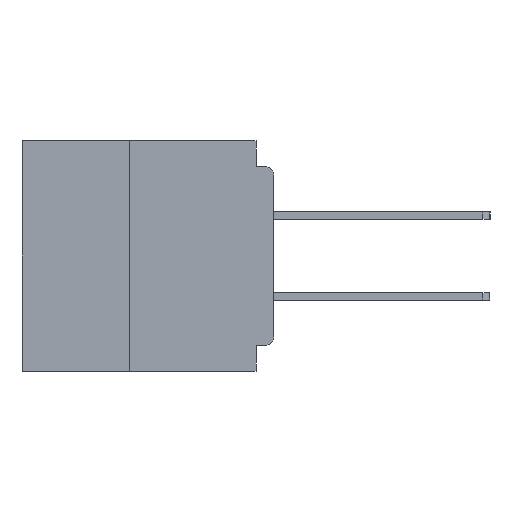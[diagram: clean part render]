
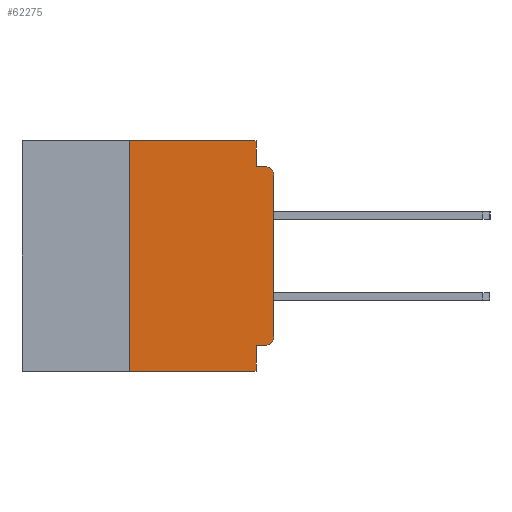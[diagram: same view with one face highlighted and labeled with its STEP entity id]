
A CAD part, left-side view. The second image highlights one B-rep face of the part: STEP entity #62275.
In plain terms, the highlighted planar face has unit normal (-1, 0, 0).
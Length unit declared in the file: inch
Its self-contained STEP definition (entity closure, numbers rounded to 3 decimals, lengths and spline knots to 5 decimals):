
#115 = LINE ( 'NONE', #27405, #37791 ) ;
#510 = CARTESIAN_POINT ( 'NONE',  ( 0., 0.031, 0. ) ) ;
#571 = VERTEX_POINT ( 'NONE', #45009 ) ;
#655 = DIRECTION ( 'NONE',  ( 0., 0., -1. ) ) ;
#2635 = ORIENTED_EDGE ( 'NONE', *, *, #33401, .T. ) ;
#2966 = CARTESIAN_POINT ( 'NONE',  ( 0., 0.437, 0. ) ) ;
#4892 = CARTESIAN_POINT ( 'NONE',  ( 0., 0.437, -0.4 ) ) ;
#5825 = EDGE_CURVE ( 'NONE', #58855, #42514, #52267, .T. ) ;
#7138 = VERTEX_POINT ( 'NONE', #64051 ) ;
#7331 = VECTOR ( 'NONE', #30076, 39.37008 ) ;
#7844 = CARTESIAN_POINT ( 'NONE',  ( 0., 0.015, -0.34 ) ) ;
#8143 = DIRECTION ( 'NONE',  ( 1., 0., 0. ) ) ;
#9761 = VECTOR ( 'NONE', #63482, 39.37008 ) ;
#10043 = DIRECTION ( 'NONE',  ( 0., -1., 0. ) ) ;
#12557 = CIRCLE ( 'NONE', #51729, 0.015 ) ;
#12967 = DIRECTION ( 'NONE',  ( 0., 0., -1. ) ) ;
#16704 = DIRECTION ( 'NONE',  ( -1., 0., 0. ) ) ;
#16877 = EDGE_CURVE ( 'NONE', #28326, #44976, #51607, .T. ) ;
#17175 = ORIENTED_EDGE ( 'NONE', *, *, #64541, .T. ) ;
#17293 = CARTESIAN_POINT ( 'NONE',  ( 0., 0., -0.355 ) ) ;
#17737 = DIRECTION ( 'NONE',  ( 0., -1., 0. ) ) ;
#18548 = CARTESIAN_POINT ( 'NONE',  ( 0., 0.015, -0.355 ) ) ;
#19412 = LINE ( 'NONE', #55279, #7331 ) ;
#19774 = EDGE_LOOP ( 'NONE', ( #2635, #41567, #21120, #51244, #49167, #52943, #44488, #63672, #28062, #17175 ) ) ;
#21120 = ORIENTED_EDGE ( 'NONE', *, *, #28034, .F. ) ;
#21624 = LINE ( 'NONE', #17293, #60496 ) ;
#22415 = DIRECTION ( 'NONE',  ( 0., 1., 0. ) ) ;
#22987 = VECTOR ( 'NONE', #10043, 39.37008 ) ;
#25151 = CARTESIAN_POINT ( 'NONE',  ( 0., 0.031, -0.355 ) ) ;
#25291 = CARTESIAN_POINT ( 'NONE',  ( 0., 0.25, -0.4 ) ) ;
#25301 = VECTOR ( 'NONE', #655, 39.37008 ) ;
#26108 = EDGE_CURVE ( 'NONE', #35972, #44976, #35428, .T. ) ;
#26579 = AXIS2_PLACEMENT_3D ( 'NONE', #2966, #8143, #43864 ) ;
#27405 = CARTESIAN_POINT ( 'NONE',  ( 0., 0.25, -0.4 ) ) ;
#27668 = LINE ( 'NONE', #46774, #53064 ) ;
#28034 = EDGE_CURVE ( 'NONE', #42514, #55253, #52552, .T. ) ;
#28062 = ORIENTED_EDGE ( 'NONE', *, *, #44499, .F. ) ;
#28326 = VERTEX_POINT ( 'NONE', #25291 ) ;
#30076 = DIRECTION ( 'NONE',  ( 0., 0., 1. ) ) ;
#31503 = VERTEX_POINT ( 'NONE', #51307 ) ;
#33401 = EDGE_CURVE ( 'NONE', #571, #31503, #19412, .T. ) ;
#33487 = CIRCLE ( 'NONE', #35390, 0.015 ) ;
#33704 = PLANE ( 'NONE',  #26579 ) ;
#35390 = AXIS2_PLACEMENT_3D ( 'NONE', #47155, #16704, #52246 ) ;
#35428 = LINE ( 'NONE', #58447, #9761 ) ;
#35972 = VERTEX_POINT ( 'NONE', #25151 ) ;
#35996 = CARTESIAN_POINT ( 'NONE',  ( 0., 0.031, -0.4 ) ) ;
#36795 = CARTESIAN_POINT ( 'NONE',  ( 0., 0.031, 0. ) ) ;
#37791 = VECTOR ( 'NONE', #42738, 39.37008 ) ;
#40332 = EDGE_CURVE ( 'NONE', #28326, #7138, #115, .T. ) ;
#41567 = ORIENTED_EDGE ( 'NONE', *, *, #57925, .T. ) ;
#42514 = VERTEX_POINT ( 'NONE', #58056 ) ;
#42738 = DIRECTION ( 'NONE',  ( 0., 0., 1. ) ) ;
#43105 = CARTESIAN_POINT ( 'NONE',  ( 0., 0., -0.045 ) ) ;
#43543 = DIRECTION ( 'NONE',  ( -1., 0., 0. ) ) ;
#43864 = DIRECTION ( 'NONE',  ( 0., 0., -1. ) ) ;
#44488 = ORIENTED_EDGE ( 'NONE', *, *, #16877, .T. ) ;
#44499 = EDGE_CURVE ( 'NONE', #55782, #35972, #21624, .T. ) ;
#44976 = VERTEX_POINT ( 'NONE', #35996 ) ;
#45009 = CARTESIAN_POINT ( 'NONE',  ( 0., 0., -0.34 ) ) ;
#46774 = CARTESIAN_POINT ( 'NONE',  ( 0., 0.437, 0. ) ) ;
#47067 = EDGE_CURVE ( 'NONE', #7138, #58855, #27668, .T. ) ;
#47155 = CARTESIAN_POINT ( 'NONE',  ( 0., 0.015, -0.06 ) ) ;
#49167 = ORIENTED_EDGE ( 'NONE', *, *, #47067, .F. ) ;
#51244 = ORIENTED_EDGE ( 'NONE', *, *, #5825, .F. ) ;
#51307 = CARTESIAN_POINT ( 'NONE',  ( 0., 0., -0.06 ) ) ;
#51607 = LINE ( 'NONE', #4892, #22987 ) ;
#51729 = AXIS2_PLACEMENT_3D ( 'NONE', #7844, #43543, #12967 ) ;
#51850 = DIRECTION ( 'NONE',  ( 0., -1., 0. ) ) ;
#52246 = DIRECTION ( 'NONE',  ( 0., 0., -1. ) ) ;
#52267 = LINE ( 'NONE', #510, #25301 ) ;
#52552 = LINE ( 'NONE', #43105, #55722 ) ;
#52943 = ORIENTED_EDGE ( 'NONE', *, *, #40332, .F. ) ;
#53064 = VECTOR ( 'NONE', #51850, 39.37008 ) ;
#55253 = VERTEX_POINT ( 'NONE', #60072 ) ;
#55279 = CARTESIAN_POINT ( 'NONE',  ( 0., 0., 0. ) ) ;
#55722 = VECTOR ( 'NONE', #17737, 39.37008 ) ;
#55782 = VERTEX_POINT ( 'NONE', #18548 ) ;
#57925 = EDGE_CURVE ( 'NONE', #31503, #55253, #33487, .T. ) ;
#58056 = CARTESIAN_POINT ( 'NONE',  ( 0., 0.031, -0.045 ) ) ;
#58447 = CARTESIAN_POINT ( 'NONE',  ( 0., 0.031, -0.4 ) ) ;
#58855 = VERTEX_POINT ( 'NONE', #36795 ) ;
#60072 = CARTESIAN_POINT ( 'NONE',  ( 0., 0.015, -0.045 ) ) ;
#60496 = VECTOR ( 'NONE', #22415, 39.37008 ) ;
#61397 = FACE_OUTER_BOUND ( 'NONE', #19774, .T. ) ;
#62275 = ADVANCED_FACE ( 'NONE', ( #61397 ), #33704, .F. ) ;
#63482 = DIRECTION ( 'NONE',  ( 0., 0., -1. ) ) ;
#63672 = ORIENTED_EDGE ( 'NONE', *, *, #26108, .F. ) ;
#64051 = CARTESIAN_POINT ( 'NONE',  ( 0., 0.25, 0. ) ) ;
#64541 = EDGE_CURVE ( 'NONE', #55782, #571, #12557, .T. ) ;
